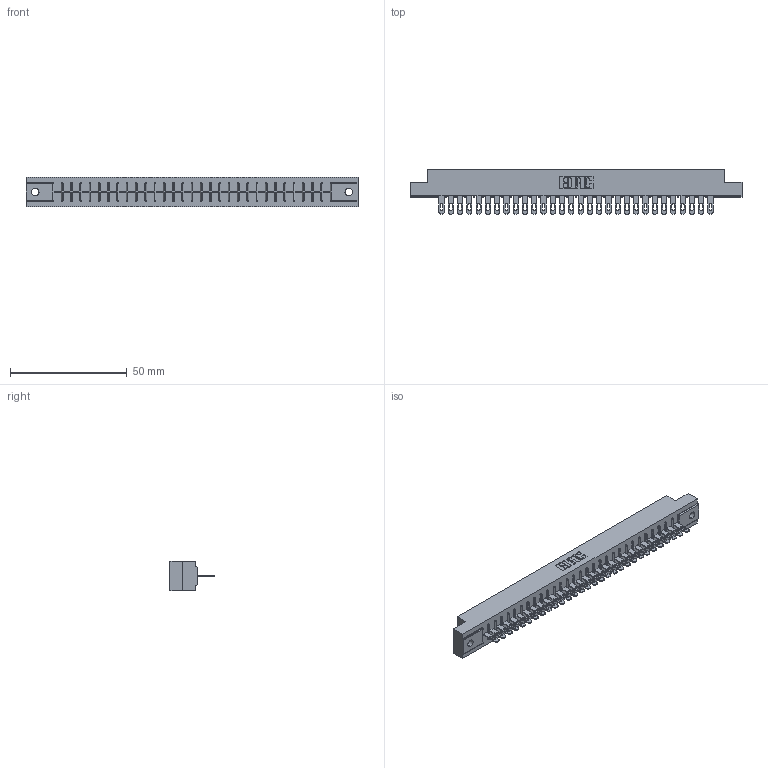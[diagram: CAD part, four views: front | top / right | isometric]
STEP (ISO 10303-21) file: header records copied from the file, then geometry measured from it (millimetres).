
FILE_DESCRIPTION (( 'STEP AP203' ), '1' );
FILE_NAME ('316-030-500-102.STEP', '2018-07-31T03:13:37', ( '' ), ( '' ), 'SwSTEP 2.0', 'SolidWorks 2016', '' );
FILE_SCHEMA (( 'CONFIG_CONTROL_DESIGN' ));
Length unit declared in the file: inch
Products named in the file (3): 306 Part_.128 Dia; 306-290-001_100; 316-030-500-102
Assembly tree (31 placements, depth 2):
  316-030-500-102
    306 Part_.128 Dia
    306-290-001_100  x30
Bounding box: 141.88 x 18.87 x 12.7 mm (x, y, z)
Volume: 15646.2 mm3; surface area: 16170.8 mm2
Topology: 31 solids, 31 shells, 2396 faces, 6766 edges, 4348 vertices
Faces by surface type: plane 1568, cylinder 708, sphere 120
Entity records: 29697 total; most frequent: CARTESIAN_POINT 4985, ORIENTED_EDGE 4940, DIRECTION 4918, EDGE_CURVE 2470, LINE 1924, VECTOR 1924, VERTEX_POINT 1564, AXIS2_PLACEMENT_3D 1497
